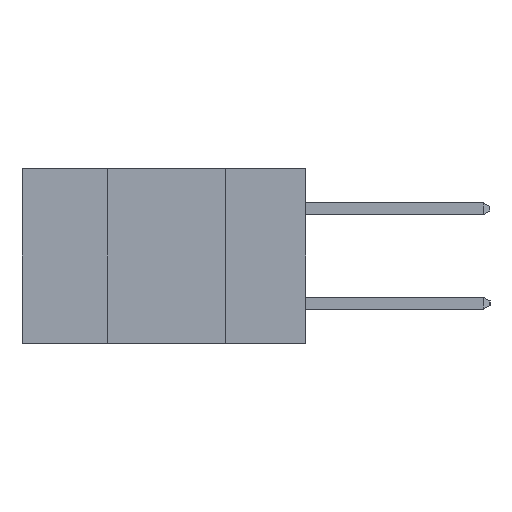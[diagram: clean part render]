
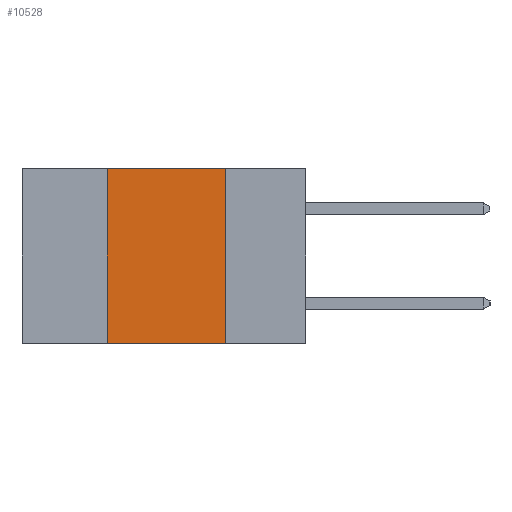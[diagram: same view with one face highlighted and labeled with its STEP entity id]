
A CAD part, left-side view. The second image highlights one B-rep face of the part: STEP entity #10528.
In plain terms, the highlighted planar face has unit normal (-1, 0, 0).
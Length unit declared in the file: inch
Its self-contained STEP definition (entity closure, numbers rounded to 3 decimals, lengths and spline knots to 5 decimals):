
#128 = ORIENTED_EDGE ( 'NONE', *, *, #343, .F. ) ;
#343 = EDGE_CURVE ( 'NONE', #1223, #11838, #3038, .T. ) ;
#793 = DIRECTION ( 'NONE',  ( 0., 0., 1. ) ) ;
#850 = AXIS2_PLACEMENT_3D ( 'NONE', #12421, #13073, #13055 ) ;
#1223 = VERTEX_POINT ( 'NONE', #7121 ) ;
#2198 = ORIENTED_EDGE ( 'NONE', *, *, #10163, .F. ) ;
#2235 = DIRECTION ( 'NONE',  ( 0., -1., 0. ) ) ;
#2597 = VECTOR ( 'NONE', #12293, 39.37008 ) ;
#2789 = VECTOR ( 'NONE', #2997, 39.37008 ) ;
#2864 = CARTESIAN_POINT ( 'NONE',  ( 0., 0.6, -0.37 ) ) ;
#2997 = DIRECTION ( 'NONE',  ( 0., -1., 0. ) ) ;
#3038 = LINE ( 'NONE', #11845, #2597 ) ;
#3117 = CARTESIAN_POINT ( 'NONE',  ( 0., 0.42, 0. ) ) ;
#4116 = ORIENTED_EDGE ( 'NONE', *, *, #9289, .T. ) ;
#4234 = VERTEX_POINT ( 'NONE', #6158 ) ;
#5842 = LINE ( 'NONE', #7522, #15469 ) ;
#6158 = CARTESIAN_POINT ( 'NONE',  ( 0., 0.42, -0.37 ) ) ;
#7031 = CARTESIAN_POINT ( 'NONE',  ( 0., 0.17, -0.37 ) ) ;
#7121 = CARTESIAN_POINT ( 'NONE',  ( 0., 0.17, 0. ) ) ;
#7522 = CARTESIAN_POINT ( 'NONE',  ( 0., 0.6, 0. ) ) ;
#9242 = VECTOR ( 'NONE', #793, 39.37008 ) ;
#9289 = EDGE_CURVE ( 'NONE', #4234, #11838, #13336, .T. ) ;
#10053 = FACE_OUTER_BOUND ( 'NONE', #10654, .T. ) ;
#10069 = LINE ( 'NONE', #14774, #9242 ) ;
#10163 = EDGE_CURVE ( 'NONE', #4234, #12316, #10069, .T. ) ;
#10528 = ADVANCED_FACE ( 'NONE', ( #10053 ), #12963, .F. ) ;
#10654 = EDGE_LOOP ( 'NONE', ( #128, #10969, #2198, #4116 ) ) ;
#10969 = ORIENTED_EDGE ( 'NONE', *, *, #14879, .F. ) ;
#11838 = VERTEX_POINT ( 'NONE', #7031 ) ;
#11845 = CARTESIAN_POINT ( 'NONE',  ( 0., 0.17, -0.37 ) ) ;
#12293 = DIRECTION ( 'NONE',  ( 0., 0., -1. ) ) ;
#12316 = VERTEX_POINT ( 'NONE', #3117 ) ;
#12421 = CARTESIAN_POINT ( 'NONE',  ( 0., 0.6, 0. ) ) ;
#12963 = PLANE ( 'NONE',  #850 ) ;
#13055 = DIRECTION ( 'NONE',  ( 0., 0., -1. ) ) ;
#13073 = DIRECTION ( 'NONE',  ( 1., 0., 0. ) ) ;
#13336 = LINE ( 'NONE', #2864, #2789 ) ;
#14774 = CARTESIAN_POINT ( 'NONE',  ( 0., 0.42, -0.37 ) ) ;
#14879 = EDGE_CURVE ( 'NONE', #12316, #1223, #5842, .T. ) ;
#15469 = VECTOR ( 'NONE', #2235, 39.37008 ) ;
